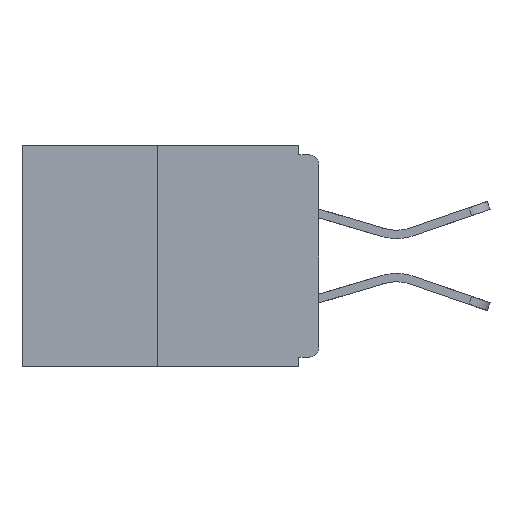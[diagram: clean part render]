
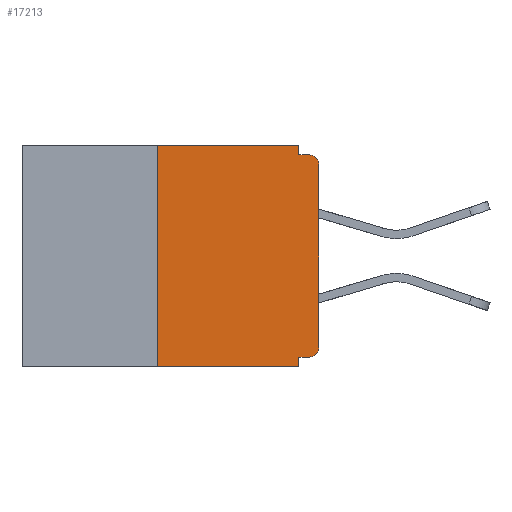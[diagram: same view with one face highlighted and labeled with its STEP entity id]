
A CAD part, left-side view. The second image highlights one B-rep face of the part: STEP entity #17213.
In plain terms, the highlighted planar face has unit normal (-1, 0, 0).
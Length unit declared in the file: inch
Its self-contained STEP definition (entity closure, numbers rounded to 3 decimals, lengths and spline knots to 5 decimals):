
#25 = DIRECTION ( 'NONE',  ( 0., 0., -1. ) ) ;
#127 = LINE ( 'NONE', #4488, #9883 ) ;
#161 = LINE ( 'NONE', #16214, #3572 ) ;
#418 = CARTESIAN_POINT ( 'NONE',  ( 0., 0.031, -0.015 ) ) ;
#496 = LINE ( 'NONE', #3390, #17005 ) ;
#712 = VERTEX_POINT ( 'NONE', #2174 ) ;
#1441 = CARTESIAN_POINT ( 'NONE',  ( 0., 0.46, 0. ) ) ;
#1749 = LINE ( 'NONE', #6219, #16782 ) ;
#1778 = EDGE_CURVE ( 'NONE', #12355, #5670, #11587, .T. ) ;
#1821 = CIRCLE ( 'NONE', #5499, 0.015 ) ;
#1921 = DIRECTION ( 'NONE',  ( -1., 0., 0. ) ) ;
#1978 = EDGE_LOOP ( 'NONE', ( #15374, #12832, #7656, #14449, #5148, #4055, #4358, #10803, #10764, #9971 ) ) ;
#2174 = CARTESIAN_POINT ( 'NONE',  ( 0., 0.031, -0.328 ) ) ;
#2628 = VERTEX_POINT ( 'NONE', #11355 ) ;
#2785 = CARTESIAN_POINT ( 'NONE',  ( 0., 0.015, -0.015 ) ) ;
#2813 = DIRECTION ( 'NONE',  ( 1., 0., 0. ) ) ;
#3090 = CIRCLE ( 'NONE', #7454, 0.015 ) ;
#3390 = CARTESIAN_POINT ( 'NONE',  ( 0., 0.25, 0. ) ) ;
#3572 = VECTOR ( 'NONE', #5385, 39.37008 ) ;
#3669 = EDGE_CURVE ( 'NONE', #17270, #12355, #496, .T. ) ;
#4055 = ORIENTED_EDGE ( 'NONE', *, *, #10908, .T. ) ;
#4317 = PLANE ( 'NONE',  #10237 ) ;
#4358 = ORIENTED_EDGE ( 'NONE', *, *, #8792, .T. ) ;
#4422 = DIRECTION ( 'NONE',  ( -1., 0., 0. ) ) ;
#4488 = CARTESIAN_POINT ( 'NONE',  ( 0., 0., -0.015 ) ) ;
#4668 = CARTESIAN_POINT ( 'NONE',  ( 0., 0.25, -0.343 ) ) ;
#4781 = DIRECTION ( 'NONE',  ( 0., 0., 1. ) ) ;
#5060 = EDGE_CURVE ( 'NONE', #712, #10218, #1749, .T. ) ;
#5148 = ORIENTED_EDGE ( 'NONE', *, *, #10011, .F. ) ;
#5385 = DIRECTION ( 'NONE',  ( 0., 0., -1. ) ) ;
#5499 = AXIS2_PLACEMENT_3D ( 'NONE', #7237, #4422, #5774 ) ;
#5670 = VERTEX_POINT ( 'NONE', #8779 ) ;
#5774 = DIRECTION ( 'NONE',  ( 0., 0., -1. ) ) ;
#5976 = CARTESIAN_POINT ( 'NONE',  ( 0., 0.015, -0.313 ) ) ;
#6084 = VECTOR ( 'NONE', #8901, 39.37008 ) ;
#6219 = CARTESIAN_POINT ( 'NONE',  ( 0., 0.031, -0.343 ) ) ;
#6309 = DIRECTION ( 'NONE',  ( 0., 0., 1. ) ) ;
#6943 = LINE ( 'NONE', #13420, #7157 ) ;
#7112 = FACE_OUTER_BOUND ( 'NONE', #1978, .T. ) ;
#7157 = VECTOR ( 'NONE', #13481, 39.37008 ) ;
#7237 = CARTESIAN_POINT ( 'NONE',  ( 0., 0.015, -0.03 ) ) ;
#7454 = AXIS2_PLACEMENT_3D ( 'NONE', #5976, #1921, #9970 ) ;
#7656 = ORIENTED_EDGE ( 'NONE', *, *, #14121, .T. ) ;
#8779 = CARTESIAN_POINT ( 'NONE',  ( 0., 0.031, 0. ) ) ;
#8792 = EDGE_CURVE ( 'NONE', #12393, #2628, #16261, .T. ) ;
#8817 = LINE ( 'NONE', #16986, #6084 ) ;
#8901 = DIRECTION ( 'NONE',  ( 0., -1., 0. ) ) ;
#9115 = CARTESIAN_POINT ( 'NONE',  ( 0., 0., 0. ) ) ;
#9591 = CARTESIAN_POINT ( 'NONE',  ( 0., 0.031, -0.343 ) ) ;
#9883 = VECTOR ( 'NONE', #10234, 39.37008 ) ;
#9970 = DIRECTION ( 'NONE',  ( 0., 0., -1. ) ) ;
#9971 = ORIENTED_EDGE ( 'NONE', *, *, #13113, .F. ) ;
#10011 = EDGE_CURVE ( 'NONE', #16811, #712, #6943, .T. ) ;
#10218 = VERTEX_POINT ( 'NONE', #9591 ) ;
#10234 = DIRECTION ( 'NONE',  ( 0., -1., 0. ) ) ;
#10237 = AXIS2_PLACEMENT_3D ( 'NONE', #1441, #2813, #25 ) ;
#10745 = CARTESIAN_POINT ( 'NONE',  ( 0., 0., -0.313 ) ) ;
#10764 = ORIENTED_EDGE ( 'NONE', *, *, #16561, .F. ) ;
#10803 = ORIENTED_EDGE ( 'NONE', *, *, #16486, .T. ) ;
#10908 = EDGE_CURVE ( 'NONE', #16811, #12393, #3090, .T. ) ;
#11166 = CARTESIAN_POINT ( 'NONE',  ( 0., 0.46, 0. ) ) ;
#11278 = DIRECTION ( 'NONE',  ( 0., -1., 0. ) ) ;
#11355 = CARTESIAN_POINT ( 'NONE',  ( 0., 0., -0.03 ) ) ;
#11587 = LINE ( 'NONE', #11166, #16666 ) ;
#12087 = VERTEX_POINT ( 'NONE', #2785 ) ;
#12258 = VECTOR ( 'NONE', #6309, 39.37008 ) ;
#12355 = VERTEX_POINT ( 'NONE', #13347 ) ;
#12393 = VERTEX_POINT ( 'NONE', #10745 ) ;
#12711 = DIRECTION ( 'NONE',  ( 0., 0., -1. ) ) ;
#12832 = ORIENTED_EDGE ( 'NONE', *, *, #3669, .F. ) ;
#12888 = VERTEX_POINT ( 'NONE', #418 ) ;
#13113 = EDGE_CURVE ( 'NONE', #5670, #12888, #161, .T. ) ;
#13347 = CARTESIAN_POINT ( 'NONE',  ( 0., 0.25, 0. ) ) ;
#13420 = CARTESIAN_POINT ( 'NONE',  ( 0., 0., -0.328 ) ) ;
#13481 = DIRECTION ( 'NONE',  ( 0., 1., 0. ) ) ;
#13867 = CARTESIAN_POINT ( 'NONE',  ( 0., 0.015, -0.328 ) ) ;
#14121 = EDGE_CURVE ( 'NONE', #17270, #10218, #8817, .T. ) ;
#14449 = ORIENTED_EDGE ( 'NONE', *, *, #5060, .F. ) ;
#15374 = ORIENTED_EDGE ( 'NONE', *, *, #1778, .F. ) ;
#16214 = CARTESIAN_POINT ( 'NONE',  ( 0., 0.031, 0. ) ) ;
#16261 = LINE ( 'NONE', #9115, #12258 ) ;
#16486 = EDGE_CURVE ( 'NONE', #2628, #12087, #1821, .T. ) ;
#16561 = EDGE_CURVE ( 'NONE', #12888, #12087, #127, .T. ) ;
#16666 = VECTOR ( 'NONE', #11278, 39.37008 ) ;
#16782 = VECTOR ( 'NONE', #12711, 39.37008 ) ;
#16811 = VERTEX_POINT ( 'NONE', #13867 ) ;
#16986 = CARTESIAN_POINT ( 'NONE',  ( 0., 0.46, -0.343 ) ) ;
#17005 = VECTOR ( 'NONE', #4781, 39.37008 ) ;
#17213 = ADVANCED_FACE ( 'NONE', ( #7112 ), #4317, .F. ) ;
#17270 = VERTEX_POINT ( 'NONE', #4668 ) ;
